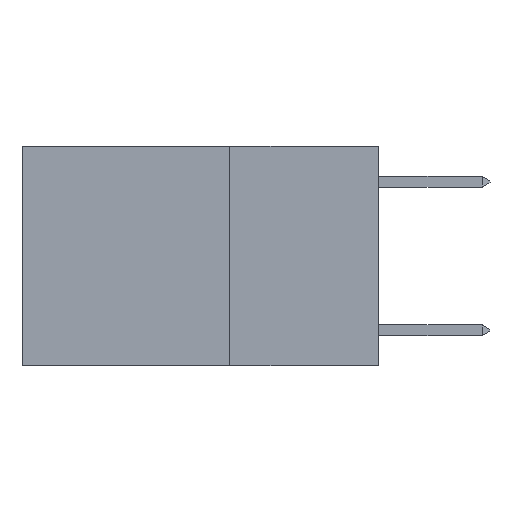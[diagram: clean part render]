
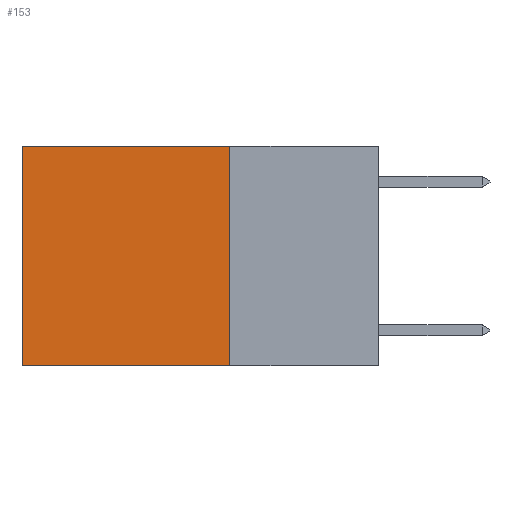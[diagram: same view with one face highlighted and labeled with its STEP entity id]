
A CAD part, left-side view. The second image highlights one B-rep face of the part: STEP entity #153.
In plain terms, the highlighted planar face has unit normal (-1, 0, 0).
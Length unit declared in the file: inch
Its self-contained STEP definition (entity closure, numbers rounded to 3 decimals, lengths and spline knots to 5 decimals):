
#153 = ADVANCED_FACE ( 'NONE', ( #1323 ), #2472, .F. ) ;
#554 = CARTESIAN_POINT ( 'NONE',  ( 0.2625, 0.6, -0.37 ) ) ;
#584 = ORIENTED_EDGE ( 'NONE', *, *, #719, .T. ) ;
#719 = EDGE_CURVE ( 'NONE', #6398, #3240, #7241, .T. ) ;
#740 = VECTOR ( 'NONE', #8175, 39.37008 ) ;
#760 = ORIENTED_EDGE ( 'NONE', *, *, #3252, .F. ) ;
#832 = CARTESIAN_POINT ( 'NONE',  ( 0.2625, 0.25, 0. ) ) ;
#1323 = FACE_OUTER_BOUND ( 'NONE', #4255, .T. ) ;
#1573 = VERTEX_POINT ( 'NONE', #832 ) ;
#1695 = VERTEX_POINT ( 'NONE', #4903 ) ;
#1974 = CARTESIAN_POINT ( 'NONE',  ( 0.2625, 0.6, 0. ) ) ;
#2077 = LINE ( 'NONE', #4870, #7132 ) ;
#2159 = VECTOR ( 'NONE', #4942, 39.37008 ) ;
#2202 = DIRECTION ( 'NONE',  ( 1., 0., 0. ) ) ;
#2339 = DIRECTION ( 'NONE',  ( 0., 1., 0. ) ) ;
#2472 = PLANE ( 'NONE',  #7724 ) ;
#3240 = VERTEX_POINT ( 'NONE', #554 ) ;
#3252 = EDGE_CURVE ( 'NONE', #1573, #1695, #2077, .T. ) ;
#3525 = CARTESIAN_POINT ( 'NONE',  ( 0.2625, 0.25, 0. ) ) ;
#3992 = VECTOR ( 'NONE', #2339, 39.37008 ) ;
#4255 = EDGE_LOOP ( 'NONE', ( #584, #4588, #760, #4447 ) ) ;
#4447 = ORIENTED_EDGE ( 'NONE', *, *, #5704, .T. ) ;
#4588 = ORIENTED_EDGE ( 'NONE', *, *, #7196, .F. ) ;
#4870 = CARTESIAN_POINT ( 'NONE',  ( 0.2625, 0.25, 0. ) ) ;
#4903 = CARTESIAN_POINT ( 'NONE',  ( 0.2625, 0.25, -0.37 ) ) ;
#4942 = DIRECTION ( 'NONE',  ( 0., 0., -1. ) ) ;
#5704 = EDGE_CURVE ( 'NONE', #1573, #6398, #5853, .T. ) ;
#5853 = LINE ( 'NONE', #7539, #740 ) ;
#5947 = LINE ( 'NONE', #6117, #3992 ) ;
#6117 = CARTESIAN_POINT ( 'NONE',  ( 0.2625, 0.25, -0.37 ) ) ;
#6398 = VERTEX_POINT ( 'NONE', #6694 ) ;
#6643 = DIRECTION ( 'NONE',  ( 0., 0., -1. ) ) ;
#6694 = CARTESIAN_POINT ( 'NONE',  ( 0.2625, 0.6, 0. ) ) ;
#7132 = VECTOR ( 'NONE', #7852, 39.37008 ) ;
#7196 = EDGE_CURVE ( 'NONE', #1695, #3240, #5947, .T. ) ;
#7241 = LINE ( 'NONE', #1974, #2159 ) ;
#7539 = CARTESIAN_POINT ( 'NONE',  ( 0.2625, 0.25, 0. ) ) ;
#7724 = AXIS2_PLACEMENT_3D ( 'NONE', #3525, #2202, #6643 ) ;
#7852 = DIRECTION ( 'NONE',  ( 0., 0., -1. ) ) ;
#8175 = DIRECTION ( 'NONE',  ( 0., 1., 0. ) ) ;
